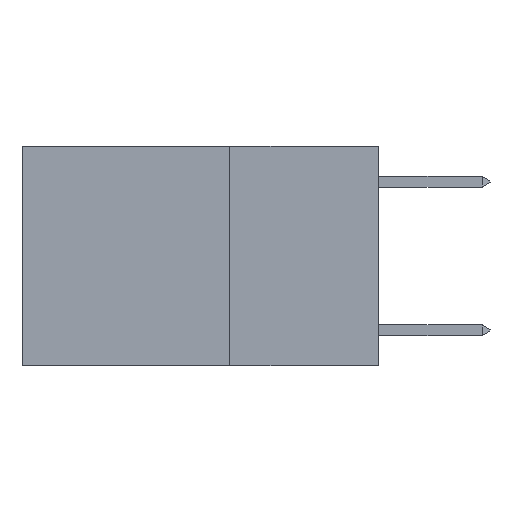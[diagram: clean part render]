
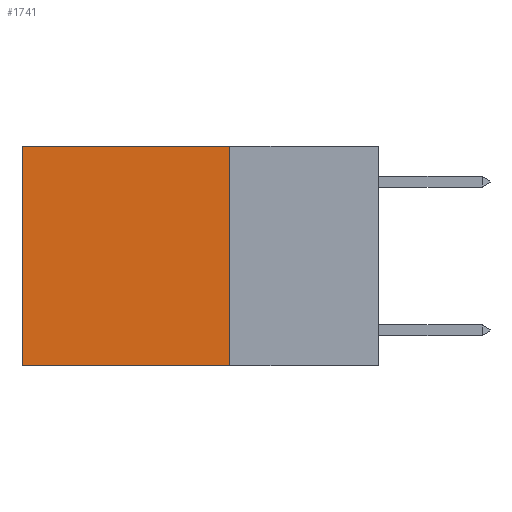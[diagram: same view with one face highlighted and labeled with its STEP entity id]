
A CAD part, left-side view. The second image highlights one B-rep face of the part: STEP entity #1741.
In plain terms, the highlighted planar face has unit normal (-1, 0, 0).
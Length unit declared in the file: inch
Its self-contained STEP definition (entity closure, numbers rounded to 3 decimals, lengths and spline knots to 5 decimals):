
#259 = VECTOR ( 'NONE', #9125, 39.37008 ) ;
#405 = VERTEX_POINT ( 'NONE', #7350 ) ;
#720 = EDGE_CURVE ( 'NONE', #7181, #405, #1665, .T. ) ;
#1393 = CARTESIAN_POINT ( 'NONE',  ( 0.2625, 0.6, 0. ) ) ;
#1451 = CARTESIAN_POINT ( 'NONE',  ( 0.2625, 0.6, 0. ) ) ;
#1598 = CARTESIAN_POINT ( 'NONE',  ( 0.2625, 0.25, 0. ) ) ;
#1665 = LINE ( 'NONE', #1393, #7018 ) ;
#1741 = ADVANCED_FACE ( 'NONE', ( #7443 ), #3257, .F. ) ;
#1962 = LINE ( 'NONE', #8763, #5685 ) ;
#2340 = ORIENTED_EDGE ( 'NONE', *, *, #7713, .F. ) ;
#2464 = DIRECTION ( 'NONE',  ( 0., 0., -1. ) ) ;
#3023 = VECTOR ( 'NONE', #9492, 39.37008 ) ;
#3097 = DIRECTION ( 'NONE',  ( 0., 0., -1. ) ) ;
#3257 = PLANE ( 'NONE',  #8723 ) ;
#4287 = EDGE_CURVE ( 'NONE', #4928, #7181, #9858, .T. ) ;
#4832 = CARTESIAN_POINT ( 'NONE',  ( 0.2625, 0.25, -0.37 ) ) ;
#4928 = VERTEX_POINT ( 'NONE', #9054 ) ;
#5685 = VECTOR ( 'NONE', #9551, 39.37008 ) ;
#6624 = CARTESIAN_POINT ( 'NONE',  ( 0.2625, 0.25, 0. ) ) ;
#6698 = ORIENTED_EDGE ( 'NONE', *, *, #8268, .F. ) ;
#7018 = VECTOR ( 'NONE', #2464, 39.37008 ) ;
#7181 = VERTEX_POINT ( 'NONE', #1451 ) ;
#7350 = CARTESIAN_POINT ( 'NONE',  ( 0.2625, 0.6, -0.37 ) ) ;
#7443 = FACE_OUTER_BOUND ( 'NONE', #8897, .T. ) ;
#7713 = EDGE_CURVE ( 'NONE', #4928, #9879, #1962, .T. ) ;
#8148 = ORIENTED_EDGE ( 'NONE', *, *, #4287, .T. ) ;
#8268 = EDGE_CURVE ( 'NONE', #9879, #405, #10275, .T. ) ;
#8354 = ORIENTED_EDGE ( 'NONE', *, *, #720, .T. ) ;
#8723 = AXIS2_PLACEMENT_3D ( 'NONE', #6624, #8888, #3097 ) ;
#8763 = CARTESIAN_POINT ( 'NONE',  ( 0.2625, 0.25, 0. ) ) ;
#8888 = DIRECTION ( 'NONE',  ( 1., 0., 0. ) ) ;
#8897 = EDGE_LOOP ( 'NONE', ( #8354, #6698, #2340, #8148 ) ) ;
#9054 = CARTESIAN_POINT ( 'NONE',  ( 0.2625, 0.25, 0. ) ) ;
#9125 = DIRECTION ( 'NONE',  ( 0., 1., 0. ) ) ;
#9492 = DIRECTION ( 'NONE',  ( 0., 1., 0. ) ) ;
#9543 = CARTESIAN_POINT ( 'NONE',  ( 0.2625, 0.25, -0.37 ) ) ;
#9551 = DIRECTION ( 'NONE',  ( 0., 0., -1. ) ) ;
#9858 = LINE ( 'NONE', #1598, #259 ) ;
#9879 = VERTEX_POINT ( 'NONE', #4832 ) ;
#10275 = LINE ( 'NONE', #9543, #3023 ) ;
